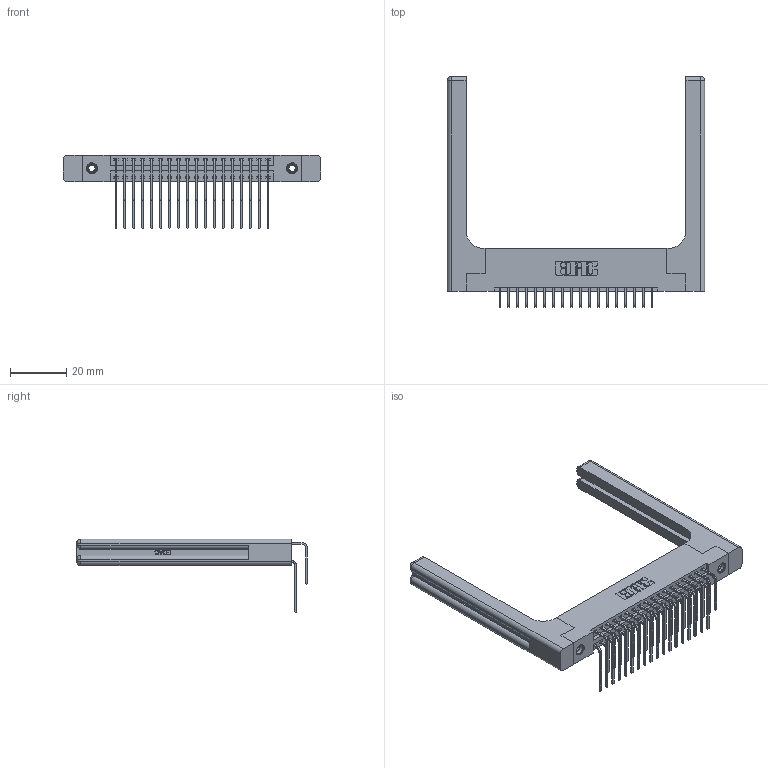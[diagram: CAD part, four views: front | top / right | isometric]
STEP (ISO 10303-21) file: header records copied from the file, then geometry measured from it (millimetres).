
FILE_DESCRIPTION (( 'STEP AP203' ), '1' );
FILE_NAME ('346-036-559-258.STEP', '2022-05-19T22:29:40', ( '' ), ( '' ), 'SwSTEP 2.0', 'SolidWorks 2020', '' );
FILE_SCHEMA (( 'CONFIG_CONTROL_DESIGN' ));
Length unit declared in the file: inch
Products named in the file (6): 345-292-001_559 Tail - 2; 345-292-001_558 559 Tail - 1; 346 Part_Flush Mounting Lugs - 0.156 Dia-TH; 346-036-559-258; 345-250-001_345-250-001-102; 346-220-058_345-220-058
Assembly tree (41 placements, depth 2):
  346-036-559-258
    346 Part_Flush Mounting Lugs - 0.156 Dia-TH
    345-292-001_558 559 Tail - 1  x18
    345-292-001_559 Tail - 2  x18
    345-250-001_345-250-001-102  x2
    346-220-058_345-220-058  x2
Bounding box: 91.21 x 81.85 x 26.16 mm (x, y, z)
Volume: 16391.7 mm3; surface area: 17856.5 mm2
Topology: 41 solids, 41 shells, 2336 faces, 6827 edges, 4482 vertices
Faces by surface type: plane 1570, cylinder 706, bspline 36, cone 12, sphere 8, torus 4
Entity records: 22360 total; most frequent: CARTESIAN_POINT 4782, ORIENTED_EDGE 3460, DIRECTION 3170, EDGE_CURVE 1730, VECTOR 1394, LINE 1394, VERTEX_POINT 1142, AXIS2_PLACEMENT_3D 888
